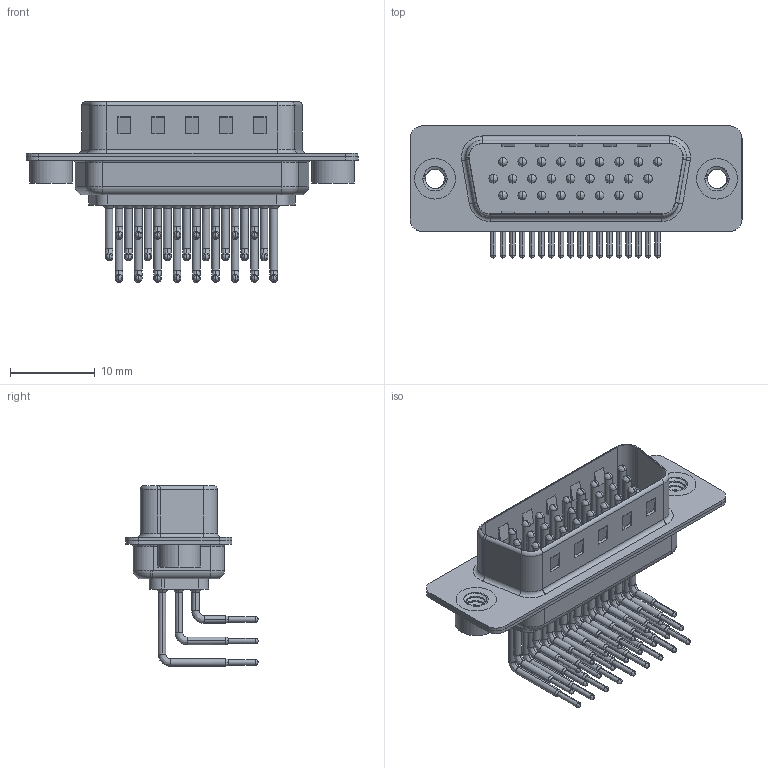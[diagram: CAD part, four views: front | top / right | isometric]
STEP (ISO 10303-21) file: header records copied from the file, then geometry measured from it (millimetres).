
FILE_DESCRIPTION (( 'STEP AP203' ), '1' );
FILE_NAME ('633-M26-363-WN2.STEP', '2018-09-27T23:16:05', ( '' ), ( '' ), 'SwSTEP 2.0', 'SolidWorks 2016', '' );
FILE_SCHEMA (( 'CONFIG_CONTROL_DESIGN' ));
Length unit declared in the file: millimetre
Products named in the file (8): 633M Contact Row 3; 633M 4-40 Threaded Rivet; 633-M26-363-WN2; 633M Housing_26 Contacts; 633M Shell Front_26 Contacts; 633M Shell Rear_26 Contacts; 633M Contact Row 1; 633M Contact Row 2
Assembly tree (31 placements, depth 2):
  633-M26-363-WN2
    633M Housing_26 Contacts
    633M Shell Front_26 Contacts
    633M Shell Rear_26 Contacts
    633M Contact Row 1  x9
    633M Contact Row 2  x9
    633M Contact Row 3  x8
    633M 4-40 Threaded Rivet  x2
Bounding box: 39.2 x 15.6 x 21.32 mm (x, y, z)
Volume: 2090.7 mm3; surface area: 6696.2 mm2
Topology: 31 solids, 31 shells, 3200 faces, 8937 edges, 5810 vertices
Faces by surface type: plane 1803, cylinder 1069, bspline 162, cone 110, torus 56
Entity records: 28495 total; most frequent: CARTESIAN_POINT 6173, DIRECTION 4549, ORIENTED_EDGE 4222, EDGE_CURVE 2111, AXIS2_PLACEMENT_3D 1653, VERTEX_POINT 1371, VECTOR 1243, LINE 1243
